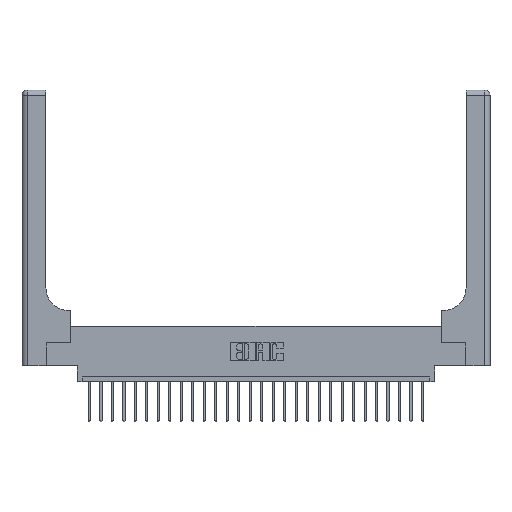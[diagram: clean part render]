
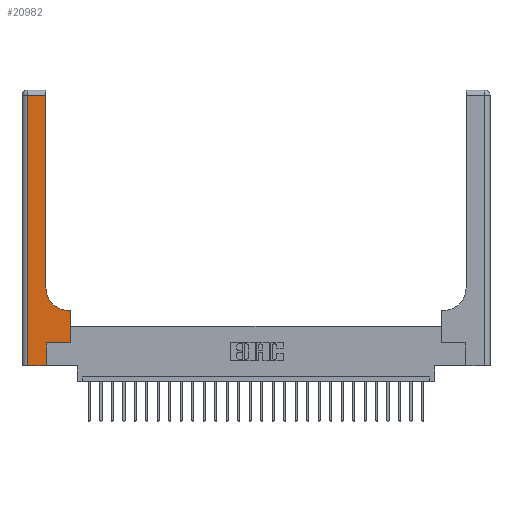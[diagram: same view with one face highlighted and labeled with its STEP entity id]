
A CAD part, top view. The second image highlights one B-rep face of the part: STEP entity #20982.
In plain terms, the highlighted planar face has unit normal (0, 0, 1).
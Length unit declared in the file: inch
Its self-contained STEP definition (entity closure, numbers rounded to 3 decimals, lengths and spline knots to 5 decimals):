
#420 = CARTESIAN_POINT ( 'NONE',  ( 0.51, 0.6, 0.37 ) ) ;
#532 = PLANE ( 'NONE',  #14802 ) ;
#721 = CARTESIAN_POINT ( 'NONE',  ( 0.265, 0.25, 0.37 ) ) ;
#1196 = ORIENTED_EDGE ( 'NONE', *, *, #6137, .T. ) ;
#1516 = EDGE_CURVE ( 'NONE', #20585, #11572, #20062, .T. ) ;
#2007 = CARTESIAN_POINT ( 'NONE',  ( 0.528, 0.6, 0.37 ) ) ;
#2139 = ORIENTED_EDGE ( 'NONE', *, *, #3707, .T. ) ;
#2591 = CARTESIAN_POINT ( 'NONE',  ( 0.528, 0.25, 0.37 ) ) ;
#2759 = LINE ( 'NONE', #14735, #15428 ) ;
#2803 = DIRECTION ( 'NONE',  ( -1., 0., 0. ) ) ;
#3077 = EDGE_CURVE ( 'NONE', #8249, #20585, #16635, .T. ) ;
#3670 = CARTESIAN_POINT ( 'NONE',  ( 0.26, 2.94, 0.37 ) ) ;
#3707 = EDGE_CURVE ( 'NONE', #15667, #9823, #18760, .T. ) ;
#4776 = LINE ( 'NONE', #12349, #14650 ) ;
#5167 = VECTOR ( 'NONE', #14055, 39.37008 ) ;
#5308 = CARTESIAN_POINT ( 'NONE',  ( 0.51, 0.85, 0.37 ) ) ;
#6137 = EDGE_CURVE ( 'NONE', #16771, #8249, #23358, .T. ) ;
#6432 = EDGE_CURVE ( 'NONE', #9823, #20658, #14427, .T. ) ;
#6614 = DIRECTION ( 'NONE',  ( 0., 0., -1. ) ) ;
#6784 = DIRECTION ( 'NONE',  ( 1., 0., 0. ) ) ;
#7259 = DIRECTION ( 'NONE',  ( 1., 0., 0. ) ) ;
#7580 = CARTESIAN_POINT ( 'NONE',  ( 0.528, 0.25, 0.37 ) ) ;
#7647 = VECTOR ( 'NONE', #23494, 39.37008 ) ;
#7705 = CARTESIAN_POINT ( 'NONE',  ( 0.265, 0., 0.37 ) ) ;
#8041 = CARTESIAN_POINT ( 'NONE',  ( 0.26, 0.85, 0.37 ) ) ;
#8249 = VERTEX_POINT ( 'NONE', #12389 ) ;
#8276 = VECTOR ( 'NONE', #17636, 39.37008 ) ;
#8895 = EDGE_CURVE ( 'NONE', #15615, #23588, #4776, .T. ) ;
#9551 = FACE_OUTER_BOUND ( 'NONE', #21980, .T. ) ;
#9823 = VERTEX_POINT ( 'NONE', #8041 ) ;
#9841 = LINE ( 'NONE', #10373, #5167 ) ;
#9885 = CARTESIAN_POINT ( 'NONE',  ( 0.06, 2.94, 0.37 ) ) ;
#10373 = CARTESIAN_POINT ( 'NONE',  ( 0., 2.94, 0.37 ) ) ;
#11572 = VERTEX_POINT ( 'NONE', #2007 ) ;
#11894 = ORIENTED_EDGE ( 'NONE', *, *, #3077, .T. ) ;
#12349 = CARTESIAN_POINT ( 'NONE',  ( 0.06, 3., 0.37 ) ) ;
#12389 = CARTESIAN_POINT ( 'NONE',  ( 0.265, 0.25, 0.37 ) ) ;
#13846 = DIRECTION ( 'NONE',  ( -1., 0., 0. ) ) ;
#14055 = DIRECTION ( 'NONE',  ( -1., 0., 0. ) ) ;
#14172 = EDGE_CURVE ( 'NONE', #20658, #15615, #9841, .T. ) ;
#14427 = LINE ( 'NONE', #19598, #8276 ) ;
#14619 = CARTESIAN_POINT ( 'NONE',  ( 0., 3., 0.37 ) ) ;
#14650 = VECTOR ( 'NONE', #18297, 39.37008 ) ;
#14735 = CARTESIAN_POINT ( 'NONE',  ( 0., 0., 0.37 ) ) ;
#14776 = LINE ( 'NONE', #21578, #21855 ) ;
#14802 = AXIS2_PLACEMENT_3D ( 'NONE', #14619, #6614, #2803 ) ;
#15428 = VECTOR ( 'NONE', #7259, 39.37008 ) ;
#15615 = VERTEX_POINT ( 'NONE', #9885 ) ;
#15667 = VERTEX_POINT ( 'NONE', #420 ) ;
#16159 = AXIS2_PLACEMENT_3D ( 'NONE', #5308, #19098, #17055 ) ;
#16401 = DIRECTION ( 'NONE',  ( 0., 1., 0. ) ) ;
#16471 = ORIENTED_EDGE ( 'NONE', *, *, #14172, .T. ) ;
#16635 = LINE ( 'NONE', #721, #18498 ) ;
#16771 = VERTEX_POINT ( 'NONE', #7705 ) ;
#17055 = DIRECTION ( 'NONE',  ( 1., 0., 0. ) ) ;
#17365 = ORIENTED_EDGE ( 'NONE', *, *, #20411, .T. ) ;
#17636 = DIRECTION ( 'NONE',  ( 0., 1., 0. ) ) ;
#18297 = DIRECTION ( 'NONE',  ( 0., -1., 0. ) ) ;
#18498 = VECTOR ( 'NONE', #6784, 39.37008 ) ;
#18760 = CIRCLE ( 'NONE', #16159, 0.25 ) ;
#18832 = ORIENTED_EDGE ( 'NONE', *, *, #8895, .T. ) ;
#19098 = DIRECTION ( 'NONE',  ( 0., 0., -1. ) ) ;
#19369 = CARTESIAN_POINT ( 'NONE',  ( 0.265, 0., 0.37 ) ) ;
#19598 = CARTESIAN_POINT ( 'NONE',  ( 0.26, 3., 0.37 ) ) ;
#20062 = LINE ( 'NONE', #2591, #21309 ) ;
#20411 = EDGE_CURVE ( 'NONE', #23588, #16771, #2759, .T. ) ;
#20585 = VERTEX_POINT ( 'NONE', #7580 ) ;
#20658 = VERTEX_POINT ( 'NONE', #3670 ) ;
#20706 = EDGE_CURVE ( 'NONE', #11572, #15667, #14776, .T. ) ;
#20982 = ADVANCED_FACE ( 'NONE', ( #9551 ), #532, .F. ) ;
#21309 = VECTOR ( 'NONE', #16401, 39.37008 ) ;
#21578 = CARTESIAN_POINT ( 'NONE',  ( 0.26, 0.6, 0.37 ) ) ;
#21855 = VECTOR ( 'NONE', #13846, 39.37008 ) ;
#21904 = CARTESIAN_POINT ( 'NONE',  ( 0.06, 0., 0.37 ) ) ;
#21980 = EDGE_LOOP ( 'NONE', ( #22958, #16471, #18832, #17365, #1196, #11894, #22707, #25015, #2139 ) ) ;
#22707 = ORIENTED_EDGE ( 'NONE', *, *, #1516, .T. ) ;
#22958 = ORIENTED_EDGE ( 'NONE', *, *, #6432, .T. ) ;
#23358 = LINE ( 'NONE', #19369, #7647 ) ;
#23494 = DIRECTION ( 'NONE',  ( 0., 1., 0. ) ) ;
#23588 = VERTEX_POINT ( 'NONE', #21904 ) ;
#25015 = ORIENTED_EDGE ( 'NONE', *, *, #20706, .T. ) ;
